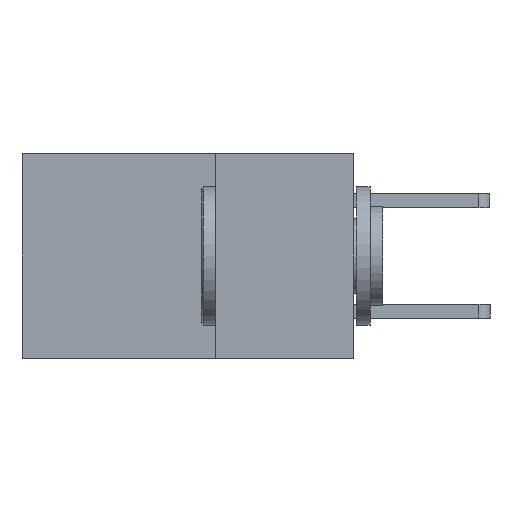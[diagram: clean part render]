
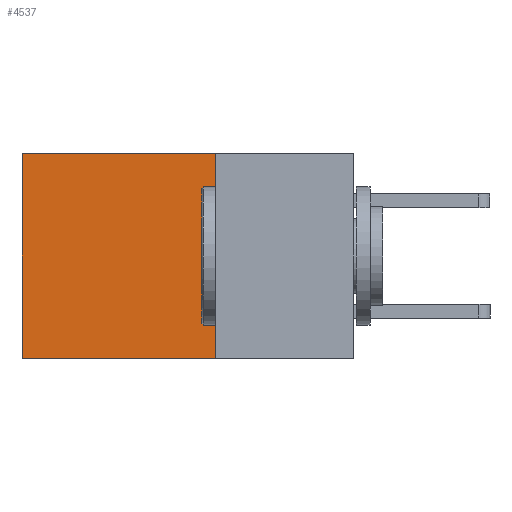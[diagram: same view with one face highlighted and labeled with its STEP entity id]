
A CAD part, left-side view. The second image highlights one B-rep face of the part: STEP entity #4537.
In plain terms, the highlighted planar face has unit normal (-1, 0, 0).
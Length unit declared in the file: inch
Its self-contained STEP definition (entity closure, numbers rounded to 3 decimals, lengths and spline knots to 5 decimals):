
#13 = PLANE ( 'NONE',  #3495 ) ;
#360 = VECTOR ( 'NONE', #10607, 39.37008 ) ;
#476 = CARTESIAN_POINT ( 'NONE',  ( 0.2875, 0.6, 0. ) ) ;
#532 = ORIENTED_EDGE ( 'NONE', *, *, #8896, .F. ) ;
#1440 = EDGE_LOOP ( 'NONE', ( #2671, #532, #2660, #9751 ) ) ;
#1607 = EDGE_CURVE ( 'NONE', #1641, #7059, #8347, .T. ) ;
#1641 = VERTEX_POINT ( 'NONE', #4962 ) ;
#1735 = CARTESIAN_POINT ( 'NONE',  ( 0.2875, 0.25, -0.37 ) ) ;
#1792 = DIRECTION ( 'NONE',  ( 0., 1., 0. ) ) ;
#2062 = LINE ( 'NONE', #3739, #8078 ) ;
#2164 = DIRECTION ( 'NONE',  ( 0., 0., -1. ) ) ;
#2397 = FACE_OUTER_BOUND ( 'NONE', #1440, .T. ) ;
#2660 = ORIENTED_EDGE ( 'NONE', *, *, #6965, .F. ) ;
#2671 = ORIENTED_EDGE ( 'NONE', *, *, #4318, .T. ) ;
#3315 = DIRECTION ( 'NONE',  ( 0., 0., -1. ) ) ;
#3495 = AXIS2_PLACEMENT_3D ( 'NONE', #5766, #10777, #3315 ) ;
#3643 = LINE ( 'NONE', #10334, #5971 ) ;
#3739 = CARTESIAN_POINT ( 'NONE',  ( 0.2875, 0.25, -0.37 ) ) ;
#4144 = CARTESIAN_POINT ( 'NONE',  ( 0.2875, 0.6, -0.37 ) ) ;
#4318 = EDGE_CURVE ( 'NONE', #7059, #5793, #6253, .T. ) ;
#4537 = ADVANCED_FACE ( 'NONE', ( #2397 ), #13, .F. ) ;
#4962 = CARTESIAN_POINT ( 'NONE',  ( 0.2875, 0.25, 0. ) ) ;
#5766 = CARTESIAN_POINT ( 'NONE',  ( 0.2875, 0.25, 0. ) ) ;
#5793 = VERTEX_POINT ( 'NONE', #4144 ) ;
#5971 = VECTOR ( 'NONE', #2164, 39.37008 ) ;
#6095 = DIRECTION ( 'NONE',  ( 0., 1., 0. ) ) ;
#6253 = LINE ( 'NONE', #476, #360 ) ;
#6965 = EDGE_CURVE ( 'NONE', #1641, #10297, #3643, .T. ) ;
#7059 = VERTEX_POINT ( 'NONE', #9883 ) ;
#8078 = VECTOR ( 'NONE', #6095, 39.37008 ) ;
#8347 = LINE ( 'NONE', #10790, #10406 ) ;
#8896 = EDGE_CURVE ( 'NONE', #10297, #5793, #2062, .T. ) ;
#9751 = ORIENTED_EDGE ( 'NONE', *, *, #1607, .T. ) ;
#9883 = CARTESIAN_POINT ( 'NONE',  ( 0.2875, 0.6, 0. ) ) ;
#10297 = VERTEX_POINT ( 'NONE', #1735 ) ;
#10334 = CARTESIAN_POINT ( 'NONE',  ( 0.2875, 0.25, 0. ) ) ;
#10406 = VECTOR ( 'NONE', #1792, 39.37008 ) ;
#10607 = DIRECTION ( 'NONE',  ( 0., 0., -1. ) ) ;
#10777 = DIRECTION ( 'NONE',  ( 1., 0., 0. ) ) ;
#10790 = CARTESIAN_POINT ( 'NONE',  ( 0.2875, 0.25, 0. ) ) ;
